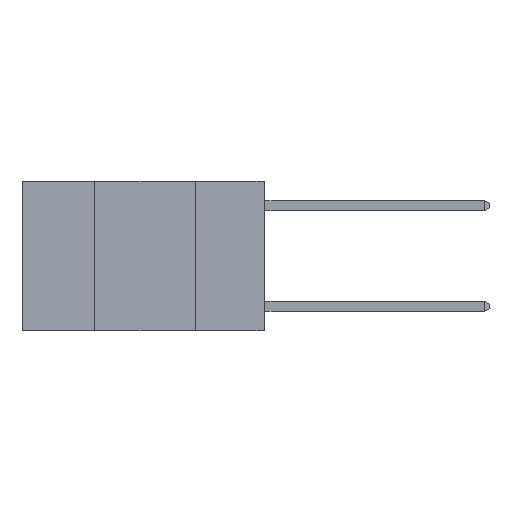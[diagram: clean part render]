
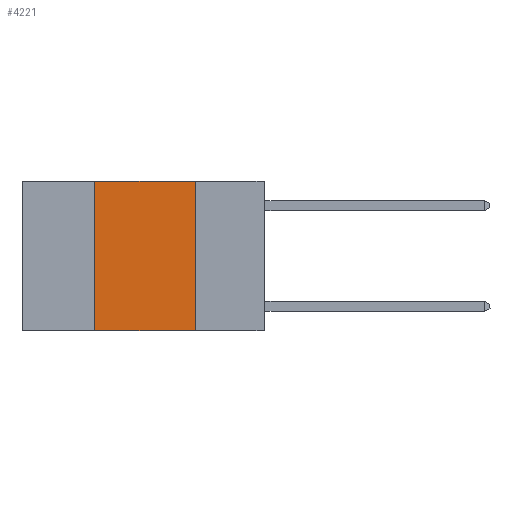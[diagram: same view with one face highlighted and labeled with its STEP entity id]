
A CAD part, left-side view. The second image highlights one B-rep face of the part: STEP entity #4221.
In plain terms, the highlighted planar face has unit normal (-1, 0, 0).
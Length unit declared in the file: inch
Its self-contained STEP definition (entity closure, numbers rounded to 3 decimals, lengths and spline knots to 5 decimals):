
#174 = EDGE_LOOP ( 'NONE', ( #5775, #5421, #8225, #1301 ) ) ;
#667 = LINE ( 'NONE', #2233, #8426 ) ;
#710 = DIRECTION ( 'NONE',  ( 0., -1., 0. ) ) ;
#1016 = VERTEX_POINT ( 'NONE', #1912 ) ;
#1296 = DIRECTION ( 'NONE',  ( 0., -1., 0. ) ) ;
#1301 = ORIENTED_EDGE ( 'NONE', *, *, #5281, .T. ) ;
#1369 = DIRECTION ( 'NONE',  ( 0., 0., 1. ) ) ;
#1405 = VERTEX_POINT ( 'NONE', #2381 ) ;
#1912 = CARTESIAN_POINT ( 'NONE',  ( 0., 0.17, 0. ) ) ;
#2108 = LINE ( 'NONE', #2150, #7930 ) ;
#2150 = CARTESIAN_POINT ( 'NONE',  ( 0., 0.17, 0. ) ) ;
#2233 = CARTESIAN_POINT ( 'NONE',  ( 0., 0.6, -0.37 ) ) ;
#2309 = FACE_OUTER_BOUND ( 'NONE', #174, .T. ) ;
#2349 = CARTESIAN_POINT ( 'NONE',  ( 0., 0.6, 0. ) ) ;
#2381 = CARTESIAN_POINT ( 'NONE',  ( 0., 0.42, 0. ) ) ;
#2805 = EDGE_CURVE ( 'NONE', #1016, #5354, #2108, .T. ) ;
#4173 = CARTESIAN_POINT ( 'NONE',  ( 0., 0.42, 0. ) ) ;
#4221 = ADVANCED_FACE ( 'NONE', ( #2309 ), #5740, .F. ) ;
#4516 = EDGE_CURVE ( 'NONE', #8038, #1405, #4693, .T. ) ;
#4693 = LINE ( 'NONE', #4173, #5829 ) ;
#5081 = DIRECTION ( 'NONE',  ( 1., 0., 0. ) ) ;
#5281 = EDGE_CURVE ( 'NONE', #8038, #5354, #667, .T. ) ;
#5354 = VERTEX_POINT ( 'NONE', #5782 ) ;
#5391 = LINE ( 'NONE', #8105, #6694 ) ;
#5421 = ORIENTED_EDGE ( 'NONE', *, *, #7716, .F. ) ;
#5740 = PLANE ( 'NONE',  #8134 ) ;
#5775 = ORIENTED_EDGE ( 'NONE', *, *, #2805, .F. ) ;
#5782 = CARTESIAN_POINT ( 'NONE',  ( 0., 0.17, -0.37 ) ) ;
#5829 = VECTOR ( 'NONE', #1369, 39.37008 ) ;
#6694 = VECTOR ( 'NONE', #1296, 39.37008 ) ;
#7227 = CARTESIAN_POINT ( 'NONE',  ( 0., 0.42, -0.37 ) ) ;
#7716 = EDGE_CURVE ( 'NONE', #1405, #1016, #5391, .T. ) ;
#7722 = DIRECTION ( 'NONE',  ( 0., 0., -1. ) ) ;
#7930 = VECTOR ( 'NONE', #8279, 39.37008 ) ;
#8038 = VERTEX_POINT ( 'NONE', #7227 ) ;
#8105 = CARTESIAN_POINT ( 'NONE',  ( 0., 0.6, 0. ) ) ;
#8134 = AXIS2_PLACEMENT_3D ( 'NONE', #2349, #5081, #7722 ) ;
#8225 = ORIENTED_EDGE ( 'NONE', *, *, #4516, .F. ) ;
#8279 = DIRECTION ( 'NONE',  ( 0., 0., -1. ) ) ;
#8426 = VECTOR ( 'NONE', #710, 39.37008 ) ;
